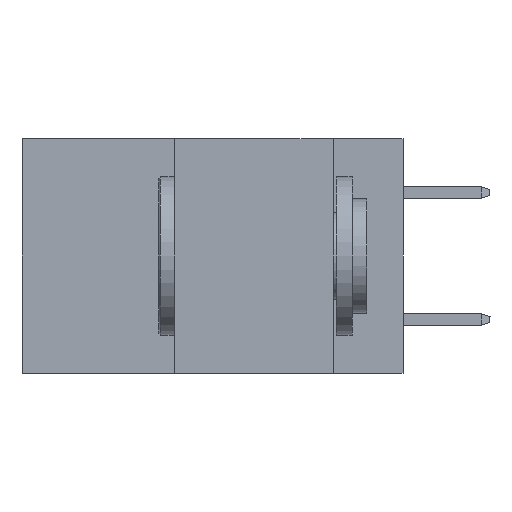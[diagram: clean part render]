
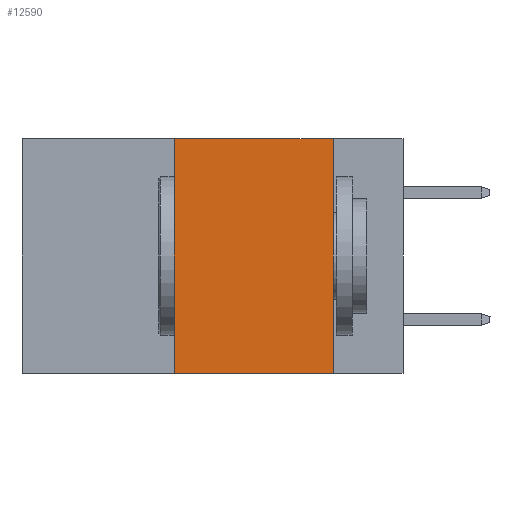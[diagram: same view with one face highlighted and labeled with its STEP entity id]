
A CAD part, left-side view. The second image highlights one B-rep face of the part: STEP entity #12590.
In plain terms, the highlighted planar face has unit normal (-1, 0, 0).
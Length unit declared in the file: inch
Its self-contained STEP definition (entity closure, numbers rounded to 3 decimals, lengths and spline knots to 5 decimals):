
#1331 = LINE ( 'NONE', #25136, #11797 ) ;
#1943 = CARTESIAN_POINT ( 'NONE',  ( 0., 0.36, -0.37 ) ) ;
#2108 = ORIENTED_EDGE ( 'NONE', *, *, #8017, .F. ) ;
#3301 = DIRECTION ( 'NONE',  ( 0., 0., -1. ) ) ;
#3934 = ORIENTED_EDGE ( 'NONE', *, *, #13120, .F. ) ;
#4521 = AXIS2_PLACEMENT_3D ( 'NONE', #27681, #17256, #3301 ) ;
#5055 = CARTESIAN_POINT ( 'NONE',  ( 0., 0.6, -0.37 ) ) ;
#7002 = CARTESIAN_POINT ( 'NONE',  ( 0., 0.11, 0. ) ) ;
#7594 = CARTESIAN_POINT ( 'NONE',  ( 0., 0.11, -0.37 ) ) ;
#7758 = CARTESIAN_POINT ( 'NONE',  ( 0., 0.36, 0. ) ) ;
#8017 = EDGE_CURVE ( 'NONE', #27485, #21575, #1331, .T. ) ;
#8391 = PLANE ( 'NONE',  #4521 ) ;
#9014 = DIRECTION ( 'NONE',  ( 0., -1., 0. ) ) ;
#9138 = VERTEX_POINT ( 'NONE', #7594 ) ;
#11797 = VECTOR ( 'NONE', #18867, 39.37008 ) ;
#12311 = VERTEX_POINT ( 'NONE', #7002 ) ;
#12590 = ADVANCED_FACE ( 'NONE', ( #28263 ), #8391, .F. ) ;
#13120 = EDGE_CURVE ( 'NONE', #12311, #9138, #19965, .T. ) ;
#13296 = CARTESIAN_POINT ( 'NONE',  ( 0., 0.11, 0. ) ) ;
#15495 = EDGE_CURVE ( 'NONE', #27485, #9138, #16091, .T. ) ;
#16091 = LINE ( 'NONE', #5055, #24150 ) ;
#16120 = VECTOR ( 'NONE', #24040, 39.37008 ) ;
#17256 = DIRECTION ( 'NONE',  ( 1., 0., 0. ) ) ;
#17685 = EDGE_CURVE ( 'NONE', #21575, #12311, #24280, .T. ) ;
#17807 = ORIENTED_EDGE ( 'NONE', *, *, #15495, .T. ) ;
#18573 = VECTOR ( 'NONE', #21410, 39.37008 ) ;
#18867 = DIRECTION ( 'NONE',  ( 0., 0., 1. ) ) ;
#19077 = EDGE_LOOP ( 'NONE', ( #3934, #23756, #2108, #17807 ) ) ;
#19965 = LINE ( 'NONE', #13296, #16120 ) ;
#21410 = DIRECTION ( 'NONE',  ( 0., -1., 0. ) ) ;
#21575 = VERTEX_POINT ( 'NONE', #7758 ) ;
#22238 = CARTESIAN_POINT ( 'NONE',  ( 0., 0.6, 0. ) ) ;
#23756 = ORIENTED_EDGE ( 'NONE', *, *, #17685, .F. ) ;
#24040 = DIRECTION ( 'NONE',  ( 0., 0., -1. ) ) ;
#24150 = VECTOR ( 'NONE', #9014, 39.37008 ) ;
#24280 = LINE ( 'NONE', #22238, #18573 ) ;
#25136 = CARTESIAN_POINT ( 'NONE',  ( 0., 0.36, 0. ) ) ;
#27485 = VERTEX_POINT ( 'NONE', #1943 ) ;
#27681 = CARTESIAN_POINT ( 'NONE',  ( 0., 0.6, 0. ) ) ;
#28263 = FACE_OUTER_BOUND ( 'NONE', #19077, .T. ) ;
